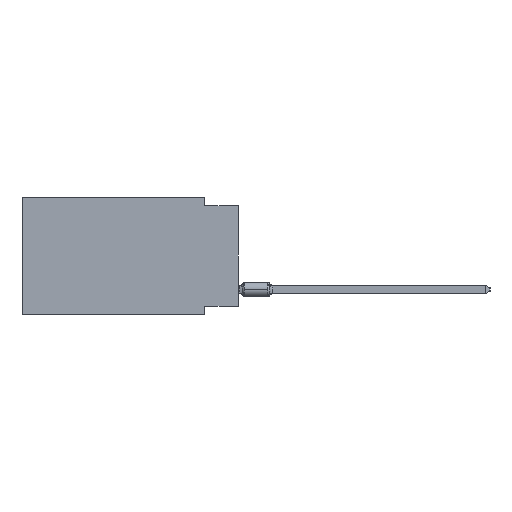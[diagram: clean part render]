
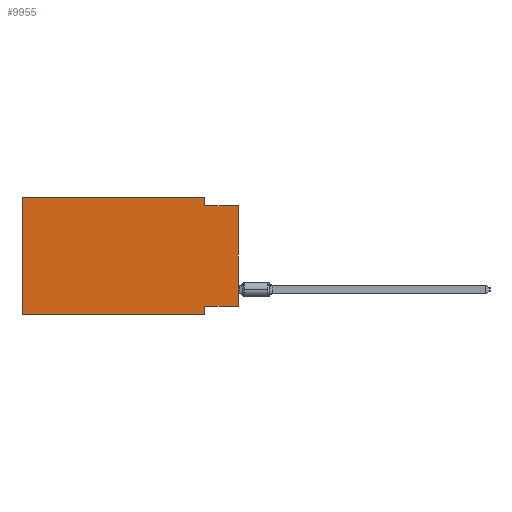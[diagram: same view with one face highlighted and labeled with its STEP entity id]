
A CAD part, left-side view. The second image highlights one B-rep face of the part: STEP entity #9955.
In plain terms, the highlighted planar face has unit normal (-1, 0, 0).
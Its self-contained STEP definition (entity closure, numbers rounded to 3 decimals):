
#294 = DIRECTION ( 'NONE',  ( 0., 0., 1. ) ) ;
#1222 = FACE_OUTER_BOUND ( 'NONE', #31124, .T. ) ;
#1499 = EDGE_CURVE ( 'NONE', #21144, #8994, #20693, .T. ) ;
#1972 = LINE ( 'NONE', #19173, #10944 ) ;
#2556 = VECTOR ( 'NONE', #30867, 1000. ) ;
#2568 = CARTESIAN_POINT ( 'NONE',  ( 0., 16.383, 0. ) ) ;
#2947 = ORIENTED_EDGE ( 'NONE', *, *, #26959, .T. ) ;
#2955 = DIRECTION ( 'NONE',  ( 0., 0., -1. ) ) ;
#3614 = DIRECTION ( 'NONE',  ( 0., -1., 0. ) ) ;
#4214 = VECTOR ( 'NONE', #294, 1000. ) ;
#4982 = EDGE_CURVE ( 'NONE', #31031, #22363, #7740, .T. ) ;
#5343 = CARTESIAN_POINT ( 'NONE',  ( 0., 2.54, -8.89 ) ) ;
#5349 = VECTOR ( 'NONE', #29948, 1000. ) ;
#5687 = CARTESIAN_POINT ( 'NONE',  ( 0., 0., -8.255 ) ) ;
#7740 = LINE ( 'NONE', #5343, #13192 ) ;
#8129 = LINE ( 'NONE', #25193, #5349 ) ;
#8369 = ORIENTED_EDGE ( 'NONE', *, *, #13678, .T. ) ;
#8536 = DIRECTION ( 'NONE',  ( 1., 0., 0. ) ) ;
#8994 = VERTEX_POINT ( 'NONE', #17507 ) ;
#9363 = CARTESIAN_POINT ( 'NONE',  ( 0., 2.54, -8.89 ) ) ;
#9955 = ADVANCED_FACE ( 'NONE', ( #1222 ), #13479, .F. ) ;
#10081 = DIRECTION ( 'NONE',  ( 0., -1., 0. ) ) ;
#10678 = ORIENTED_EDGE ( 'NONE', *, *, #27681, .F. ) ;
#10861 = ORIENTED_EDGE ( 'NONE', *, *, #4982, .F. ) ;
#10944 = VECTOR ( 'NONE', #28575, 1000. ) ;
#11087 = CARTESIAN_POINT ( 'NONE',  ( 0., 16.383, 0. ) ) ;
#11123 = CARTESIAN_POINT ( 'NONE',  ( 0., 2.54, 0. ) ) ;
#11601 = VERTEX_POINT ( 'NONE', #27508 ) ;
#12080 = CARTESIAN_POINT ( 'NONE',  ( 0., 0., -0.635 ) ) ;
#12555 = ORIENTED_EDGE ( 'NONE', *, *, #28997, .F. ) ;
#12625 = CARTESIAN_POINT ( 'NONE',  ( 0., 2.54, -8.255 ) ) ;
#13192 = VECTOR ( 'NONE', #2955, 1000. ) ;
#13479 = PLANE ( 'NONE',  #15786 ) ;
#13678 = EDGE_CURVE ( 'NONE', #16928, #22363, #18439, .T. ) ;
#15786 = AXIS2_PLACEMENT_3D ( 'NONE', #11087, #8536, #23204 ) ;
#16487 = ORIENTED_EDGE ( 'NONE', *, *, #25555, .F. ) ;
#16928 = VERTEX_POINT ( 'NONE', #26417 ) ;
#17113 = VECTOR ( 'NONE', #30060, 1000. ) ;
#17418 = CARTESIAN_POINT ( 'NONE',  ( 0., 0., -0.635 ) ) ;
#17507 = CARTESIAN_POINT ( 'NONE',  ( 0., 2.54, -0.635 ) ) ;
#18439 = LINE ( 'NONE', #20982, #22759 ) ;
#19173 = CARTESIAN_POINT ( 'NONE',  ( 0., 0., 0. ) ) ;
#20693 = LINE ( 'NONE', #11123, #2556 ) ;
#20982 = CARTESIAN_POINT ( 'NONE',  ( 0., 16.383, -8.89 ) ) ;
#21144 = VERTEX_POINT ( 'NONE', #22933 ) ;
#21611 = VERTEX_POINT ( 'NONE', #2568 ) ;
#22363 = VERTEX_POINT ( 'NONE', #9363 ) ;
#22759 = VECTOR ( 'NONE', #3614, 1000. ) ;
#22933 = CARTESIAN_POINT ( 'NONE',  ( 0., 2.54, 0. ) ) ;
#23204 = DIRECTION ( 'NONE',  ( 0., 0., -1. ) ) ;
#24057 = CARTESIAN_POINT ( 'NONE',  ( 0., 16.383, 0. ) ) ;
#24204 = LINE ( 'NONE', #24057, #4214 ) ;
#24450 = ORIENTED_EDGE ( 'NONE', *, *, #1499, .F. ) ;
#25193 = CARTESIAN_POINT ( 'NONE',  ( 0., 16.383, 0. ) ) ;
#25555 = EDGE_CURVE ( 'NONE', #16928, #21611, #24204, .T. ) ;
#25591 = VERTEX_POINT ( 'NONE', #12080 ) ;
#26391 = EDGE_CURVE ( 'NONE', #8994, #25591, #27621, .T. ) ;
#26417 = CARTESIAN_POINT ( 'NONE',  ( 0., 16.383, -8.89 ) ) ;
#26959 = EDGE_CURVE ( 'NONE', #11601, #25591, #1972, .T. ) ;
#27119 = ORIENTED_EDGE ( 'NONE', *, *, #26391, .F. ) ;
#27508 = CARTESIAN_POINT ( 'NONE',  ( 0., 0., -8.255 ) ) ;
#27516 = LINE ( 'NONE', #5687, #17113 ) ;
#27621 = LINE ( 'NONE', #17418, #29706 ) ;
#27681 = EDGE_CURVE ( 'NONE', #21611, #21144, #8129, .T. ) ;
#28575 = DIRECTION ( 'NONE',  ( 0., 0., 1. ) ) ;
#28997 = EDGE_CURVE ( 'NONE', #11601, #31031, #27516, .T. ) ;
#29706 = VECTOR ( 'NONE', #10081, 1000. ) ;
#29948 = DIRECTION ( 'NONE',  ( 0., -1., 0. ) ) ;
#30060 = DIRECTION ( 'NONE',  ( 0., 1., 0. ) ) ;
#30867 = DIRECTION ( 'NONE',  ( 0., 0., -1. ) ) ;
#31031 = VERTEX_POINT ( 'NONE', #12625 ) ;
#31124 = EDGE_LOOP ( 'NONE', ( #2947, #27119, #24450, #10678, #16487, #8369, #10861, #12555 ) ) ;
